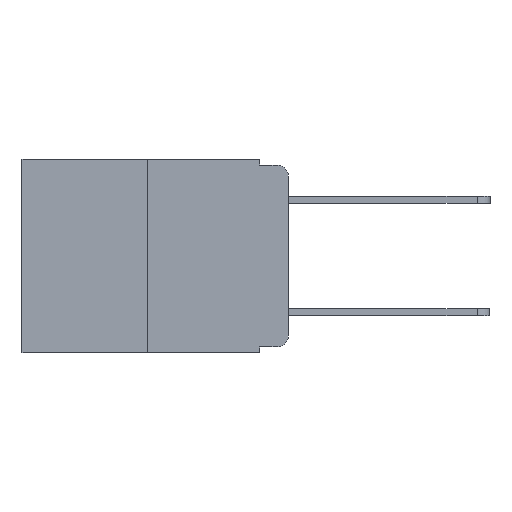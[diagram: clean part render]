
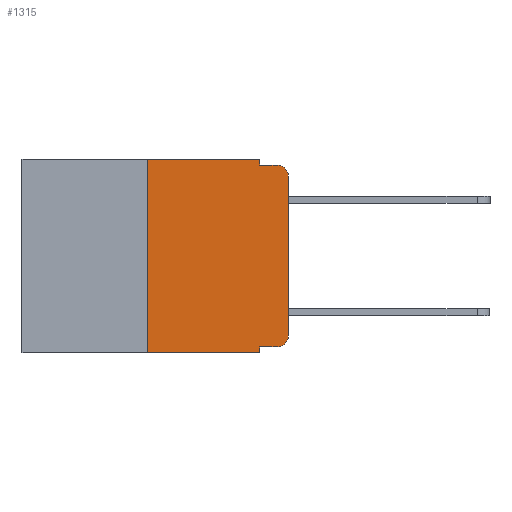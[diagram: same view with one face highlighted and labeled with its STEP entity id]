
A CAD part, left-side view. The second image highlights one B-rep face of the part: STEP entity #1315.
In plain terms, the highlighted planar face has unit normal (-1, 0, 0).
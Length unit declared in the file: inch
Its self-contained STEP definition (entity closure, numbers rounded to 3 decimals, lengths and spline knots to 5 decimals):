
#6 = EDGE_CURVE ( 'NONE', #3865, #3493, #476, .T. ) ;
#21 = ORIENTED_EDGE ( 'NONE', *, *, #10933, .F. ) ;
#63 = CIRCLE ( 'NONE', #8132, 0.02 ) ;
#476 = LINE ( 'NONE', #2509, #10230 ) ;
#645 = DIRECTION ( 'NONE',  ( 0., -1., 0. ) ) ;
#1315 = ADVANCED_FACE ( 'NONE', ( #1952 ), #3833, .F. ) ;
#1952 = FACE_OUTER_BOUND ( 'NONE', #6010, .T. ) ;
#2107 = EDGE_CURVE ( 'NONE', #9558, #5144, #8899, .T. ) ;
#2123 = LINE ( 'NONE', #6470, #4443 ) ;
#2236 = ORIENTED_EDGE ( 'NONE', *, *, #2107, .T. ) ;
#2382 = AXIS2_PLACEMENT_3D ( 'NONE', #10822, #10790, #4557 ) ;
#2419 = CARTESIAN_POINT ( 'NONE',  ( 0., 0.02, -0.333 ) ) ;
#2509 = CARTESIAN_POINT ( 'NONE',  ( 0., 0.473, 0. ) ) ;
#2516 = LINE ( 'NONE', #7269, #9049 ) ;
#2522 = DIRECTION ( 'NONE',  ( 0., 0., -1. ) ) ;
#2775 = EDGE_CURVE ( 'NONE', #12052, #9558, #11216, .T. ) ;
#3012 = VECTOR ( 'NONE', #645, 39.37008 ) ;
#3209 = VERTEX_POINT ( 'NONE', #5439 ) ;
#3493 = VERTEX_POINT ( 'NONE', #10967 ) ;
#3833 = PLANE ( 'NONE',  #2382 ) ;
#3865 = VERTEX_POINT ( 'NONE', #11334 ) ;
#3952 = CARTESIAN_POINT ( 'NONE',  ( 0., 0.051, -0.01 ) ) ;
#4372 = VECTOR ( 'NONE', #4432, 39.37008 ) ;
#4432 = DIRECTION ( 'NONE',  ( 0., 0., 1. ) ) ;
#4443 = VECTOR ( 'NONE', #10005, 39.37008 ) ;
#4557 = DIRECTION ( 'NONE',  ( 0., 0., -1. ) ) ;
#4727 = VERTEX_POINT ( 'NONE', #12107 ) ;
#4745 = DIRECTION ( 'NONE',  ( -1., 0., 0. ) ) ;
#4783 = CARTESIAN_POINT ( 'NONE',  ( 0., 0.25, 0. ) ) ;
#5049 = DIRECTION ( 'NONE',  ( 0., 0., -1. ) ) ;
#5144 = VERTEX_POINT ( 'NONE', #10122 ) ;
#5145 = VECTOR ( 'NONE', #6597, 39.37008 ) ;
#5439 = CARTESIAN_POINT ( 'NONE',  ( 0., 0.051, -0.01 ) ) ;
#5714 = ORIENTED_EDGE ( 'NONE', *, *, #9186, .T. ) ;
#5723 = VECTOR ( 'NONE', #5049, 39.37008 ) ;
#6010 = EDGE_LOOP ( 'NONE', ( #11625, #2236, #9605, #11918, #7588, #21, #7871, #10147, #5714, #8121 ) ) ;
#6041 = CARTESIAN_POINT ( 'NONE',  ( 0., 0., 0. ) ) ;
#6470 = CARTESIAN_POINT ( 'NONE',  ( 0., 0.051, -0.333 ) ) ;
#6597 = DIRECTION ( 'NONE',  ( 0., 0., 1. ) ) ;
#6793 = VERTEX_POINT ( 'NONE', #8223 ) ;
#7269 = CARTESIAN_POINT ( 'NONE',  ( 0., 0.051, 0. ) ) ;
#7468 = CARTESIAN_POINT ( 'NONE',  ( 0., 0.473, -0.343 ) ) ;
#7586 = LINE ( 'NONE', #4783, #5145 ) ;
#7588 = ORIENTED_EDGE ( 'NONE', *, *, #6, .F. ) ;
#7747 = CARTESIAN_POINT ( 'NONE',  ( 0., 0., -0.03 ) ) ;
#7871 = ORIENTED_EDGE ( 'NONE', *, *, #11646, .T. ) ;
#8121 = ORIENTED_EDGE ( 'NONE', *, *, #8633, .T. ) ;
#8132 = AXIS2_PLACEMENT_3D ( 'NONE', #10100, #4745, #10957 ) ;
#8223 = CARTESIAN_POINT ( 'NONE',  ( 0., 0.051, -0.343 ) ) ;
#8633 = EDGE_CURVE ( 'NONE', #10625, #12052, #63, .T. ) ;
#8735 = DIRECTION ( 'NONE',  ( -1., 0., 0. ) ) ;
#8748 = CARTESIAN_POINT ( 'NONE',  ( 0., 0.02, -0.03 ) ) ;
#8783 = DIRECTION ( 'NONE',  ( 0., -1., 0. ) ) ;
#8899 = CIRCLE ( 'NONE', #8937, 0.02 ) ;
#8937 = AXIS2_PLACEMENT_3D ( 'NONE', #8748, #8735, #10485 ) ;
#9049 = VECTOR ( 'NONE', #2522, 39.37008 ) ;
#9186 = EDGE_CURVE ( 'NONE', #10383, #10625, #2123, .T. ) ;
#9545 = CARTESIAN_POINT ( 'NONE',  ( 0., 0.051, -0.333 ) ) ;
#9558 = VERTEX_POINT ( 'NONE', #7747 ) ;
#9605 = ORIENTED_EDGE ( 'NONE', *, *, #12097, .F. ) ;
#10005 = DIRECTION ( 'NONE',  ( 0., -1., 0. ) ) ;
#10100 = CARTESIAN_POINT ( 'NONE',  ( 0., 0.02, -0.313 ) ) ;
#10122 = CARTESIAN_POINT ( 'NONE',  ( 0., 0.02, -0.01 ) ) ;
#10147 = ORIENTED_EDGE ( 'NONE', *, *, #10368, .F. ) ;
#10230 = VECTOR ( 'NONE', #8783, 39.37008 ) ;
#10249 = DIRECTION ( 'NONE',  ( 0., -1., 0. ) ) ;
#10279 = LINE ( 'NONE', #7468, #3012 ) ;
#10368 = EDGE_CURVE ( 'NONE', #10383, #6793, #10435, .T. ) ;
#10383 = VERTEX_POINT ( 'NONE', #9545 ) ;
#10384 = CARTESIAN_POINT ( 'NONE',  ( 0., 0.051, 0. ) ) ;
#10435 = LINE ( 'NONE', #10384, #5723 ) ;
#10485 = DIRECTION ( 'NONE',  ( 0., 0., -1. ) ) ;
#10539 = VECTOR ( 'NONE', #10249, 39.37008 ) ;
#10625 = VERTEX_POINT ( 'NONE', #2419 ) ;
#10790 = DIRECTION ( 'NONE',  ( 1., 0., 0. ) ) ;
#10812 = LINE ( 'NONE', #3952, #10539 ) ;
#10822 = CARTESIAN_POINT ( 'NONE',  ( 0., 0.473, 0. ) ) ;
#10933 = EDGE_CURVE ( 'NONE', #4727, #3865, #7586, .T. ) ;
#10957 = DIRECTION ( 'NONE',  ( 0., 0., -1. ) ) ;
#10967 = CARTESIAN_POINT ( 'NONE',  ( 0., 0.051, 0. ) ) ;
#11082 = CARTESIAN_POINT ( 'NONE',  ( 0., 0., -0.313 ) ) ;
#11216 = LINE ( 'NONE', #6041, #4372 ) ;
#11334 = CARTESIAN_POINT ( 'NONE',  ( 0., 0.25, 0. ) ) ;
#11507 = EDGE_CURVE ( 'NONE', #3493, #3209, #2516, .T. ) ;
#11625 = ORIENTED_EDGE ( 'NONE', *, *, #2775, .T. ) ;
#11646 = EDGE_CURVE ( 'NONE', #4727, #6793, #10279, .T. ) ;
#11918 = ORIENTED_EDGE ( 'NONE', *, *, #11507, .F. ) ;
#12052 = VERTEX_POINT ( 'NONE', #11082 ) ;
#12097 = EDGE_CURVE ( 'NONE', #3209, #5144, #10812, .T. ) ;
#12107 = CARTESIAN_POINT ( 'NONE',  ( 0., 0.25, -0.343 ) ) ;
